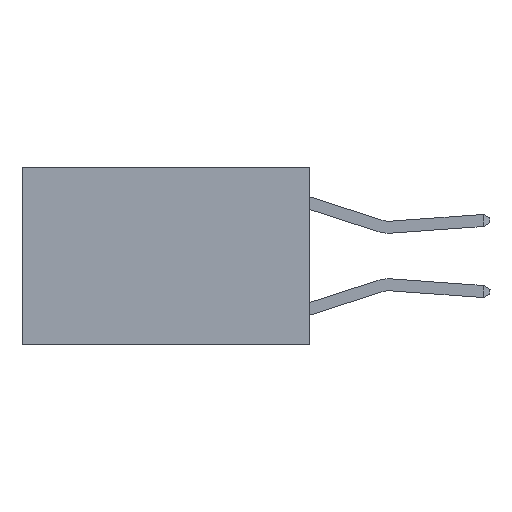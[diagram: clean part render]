
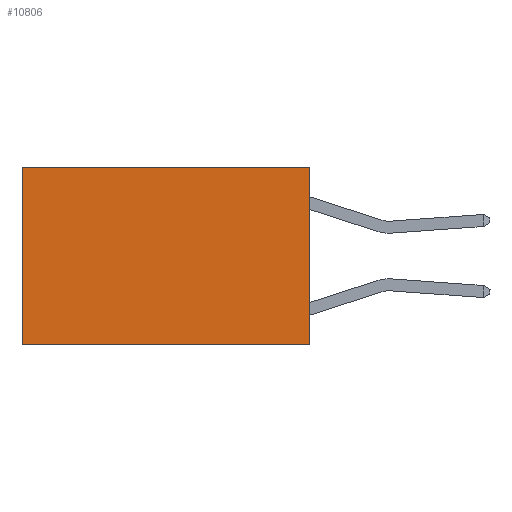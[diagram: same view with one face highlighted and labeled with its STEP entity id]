
A CAD part, left-side view. The second image highlights one B-rep face of the part: STEP entity #10806.
In plain terms, the highlighted planar face has unit normal (-1, 0, 0).
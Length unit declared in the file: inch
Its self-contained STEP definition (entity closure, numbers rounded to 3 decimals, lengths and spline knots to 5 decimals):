
#700 = DIRECTION ( 'NONE',  ( 0., 0., -1. ) ) ;
#708 = DIRECTION ( 'NONE',  ( 0., 1., 0. ) ) ;
#853 = ORIENTED_EDGE ( 'NONE', *, *, #7978, .T. ) ;
#1352 = EDGE_LOOP ( 'NONE', ( #16506, #21906, #9352, #853 ) ) ;
#2007 = VECTOR ( 'NONE', #708, 39.37008 ) ;
#2400 = CARTESIAN_POINT ( 'NONE',  ( 0.2625, 0., 0. ) ) ;
#2549 = CARTESIAN_POINT ( 'NONE',  ( 0.2625, 0., -0.37 ) ) ;
#2836 = DIRECTION ( 'NONE',  ( 1., 0., 0. ) ) ;
#3242 = AXIS2_PLACEMENT_3D ( 'NONE', #4534, #2836, #11062 ) ;
#4218 = CARTESIAN_POINT ( 'NONE',  ( 0.2625, 0., 0. ) ) ;
#4226 = EDGE_CURVE ( 'NONE', #20177, #21505, #12437, .T. ) ;
#4534 = CARTESIAN_POINT ( 'NONE',  ( 0.2625, 0., 0. ) ) ;
#5273 = VERTEX_POINT ( 'NONE', #4218 ) ;
#7978 = EDGE_CURVE ( 'NONE', #5273, #11787, #11176, .T. ) ;
#8578 = FACE_OUTER_BOUND ( 'NONE', #1352, .T. ) ;
#8952 = CARTESIAN_POINT ( 'NONE',  ( 0.2625, 0.6, 0. ) ) ;
#9352 = ORIENTED_EDGE ( 'NONE', *, *, #13501, .F. ) ;
#10806 = ADVANCED_FACE ( 'NONE', ( #8578 ), #20918, .F. ) ;
#11040 = LINE ( 'NONE', #8952, #13778 ) ;
#11062 = DIRECTION ( 'NONE',  ( 0., 0., -1. ) ) ;
#11176 = LINE ( 'NONE', #20917, #12540 ) ;
#11787 = VERTEX_POINT ( 'NONE', #12294 ) ;
#12294 = CARTESIAN_POINT ( 'NONE',  ( 0.2625, 0.6, 0. ) ) ;
#12429 = LINE ( 'NONE', #2400, #20785 ) ;
#12437 = LINE ( 'NONE', #2549, #2007 ) ;
#12540 = VECTOR ( 'NONE', #19072, 39.37008 ) ;
#13501 = EDGE_CURVE ( 'NONE', #5273, #20177, #12429, .T. ) ;
#13778 = VECTOR ( 'NONE', #16849, 39.37008 ) ;
#15916 = CARTESIAN_POINT ( 'NONE',  ( 0.2625, 0.6, -0.37 ) ) ;
#16506 = ORIENTED_EDGE ( 'NONE', *, *, #20750, .T. ) ;
#16849 = DIRECTION ( 'NONE',  ( 0., 0., -1. ) ) ;
#19072 = DIRECTION ( 'NONE',  ( 0., 1., 0. ) ) ;
#20177 = VERTEX_POINT ( 'NONE', #20821 ) ;
#20750 = EDGE_CURVE ( 'NONE', #11787, #21505, #11040, .T. ) ;
#20785 = VECTOR ( 'NONE', #700, 39.37008 ) ;
#20821 = CARTESIAN_POINT ( 'NONE',  ( 0.2625, 0., -0.37 ) ) ;
#20917 = CARTESIAN_POINT ( 'NONE',  ( 0.2625, 0., 0. ) ) ;
#20918 = PLANE ( 'NONE',  #3242 ) ;
#21505 = VERTEX_POINT ( 'NONE', #15916 ) ;
#21906 = ORIENTED_EDGE ( 'NONE', *, *, #4226, .F. ) ;
